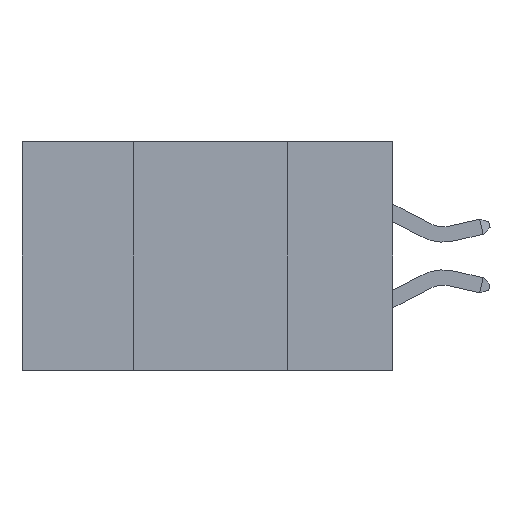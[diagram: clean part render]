
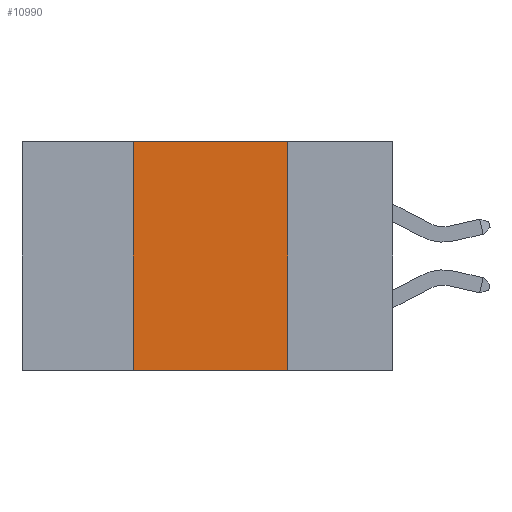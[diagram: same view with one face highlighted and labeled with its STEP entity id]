
A CAD part, left-side view. The second image highlights one B-rep face of the part: STEP entity #10990.
In plain terms, the highlighted planar face has unit normal (-1, 0, 0).
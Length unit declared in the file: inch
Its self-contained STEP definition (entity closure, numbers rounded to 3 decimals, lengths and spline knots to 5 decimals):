
#203 = CARTESIAN_POINT ( 'NONE',  ( 0., 0.17, 0. ) ) ;
#1215 = EDGE_CURVE ( 'NONE', #13711, #1265, #5261, .T. ) ;
#1265 = VERTEX_POINT ( 'NONE', #203 ) ;
#1697 = CARTESIAN_POINT ( 'NONE',  ( 0., 0.6, 0. ) ) ;
#1759 = VECTOR ( 'NONE', #15544, 39.37008 ) ;
#1935 = EDGE_CURVE ( 'NONE', #15749, #13120, #14973, .T. ) ;
#2468 = CARTESIAN_POINT ( 'NONE',  ( 0., 0.17, 0. ) ) ;
#2548 = CARTESIAN_POINT ( 'NONE',  ( 0., 0.6, -0.37 ) ) ;
#3138 = DIRECTION ( 'NONE',  ( 1., 0., 0. ) ) ;
#3873 = DIRECTION ( 'NONE',  ( 0., 0., -1. ) ) ;
#4682 = CARTESIAN_POINT ( 'NONE',  ( 0., 0.42, 0. ) ) ;
#5261 = LINE ( 'NONE', #16892, #13808 ) ;
#5322 = CARTESIAN_POINT ( 'NONE',  ( 0., 0.42, 0. ) ) ;
#5934 = LINE ( 'NONE', #5322, #1759 ) ;
#6171 = FACE_OUTER_BOUND ( 'NONE', #10884, .T. ) ;
#6976 = EDGE_CURVE ( 'NONE', #1265, #13120, #14446, .T. ) ;
#7239 = PLANE ( 'NONE',  #12774 ) ;
#8627 = DIRECTION ( 'NONE',  ( 0., -1., 0. ) ) ;
#10445 = ORIENTED_EDGE ( 'NONE', *, *, #6976, .F. ) ;
#10654 = ORIENTED_EDGE ( 'NONE', *, *, #1215, .F. ) ;
#10739 = ORIENTED_EDGE ( 'NONE', *, *, #11622, .F. ) ;
#10884 = EDGE_LOOP ( 'NONE', ( #10445, #10654, #10739, #10902 ) ) ;
#10902 = ORIENTED_EDGE ( 'NONE', *, *, #1935, .T. ) ;
#10990 = ADVANCED_FACE ( 'NONE', ( #6171 ), #7239, .F. ) ;
#11163 = VECTOR ( 'NONE', #3873, 39.37008 ) ;
#11287 = CARTESIAN_POINT ( 'NONE',  ( 0., 0.17, -0.37 ) ) ;
#11587 = DIRECTION ( 'NONE',  ( 0., -1., 0. ) ) ;
#11622 = EDGE_CURVE ( 'NONE', #15749, #13711, #5934, .T. ) ;
#12400 = DIRECTION ( 'NONE',  ( 0., 0., -1. ) ) ;
#12774 = AXIS2_PLACEMENT_3D ( 'NONE', #1697, #3138, #12400 ) ;
#13120 = VERTEX_POINT ( 'NONE', #11287 ) ;
#13711 = VERTEX_POINT ( 'NONE', #4682 ) ;
#13808 = VECTOR ( 'NONE', #11587, 39.37008 ) ;
#14446 = LINE ( 'NONE', #2468, #11163 ) ;
#14584 = VECTOR ( 'NONE', #8627, 39.37008 ) ;
#14973 = LINE ( 'NONE', #2548, #14584 ) ;
#15544 = DIRECTION ( 'NONE',  ( 0., 0., 1. ) ) ;
#15749 = VERTEX_POINT ( 'NONE', #16347 ) ;
#16347 = CARTESIAN_POINT ( 'NONE',  ( 0., 0.42, -0.37 ) ) ;
#16892 = CARTESIAN_POINT ( 'NONE',  ( 0., 0.6, 0. ) ) ;
